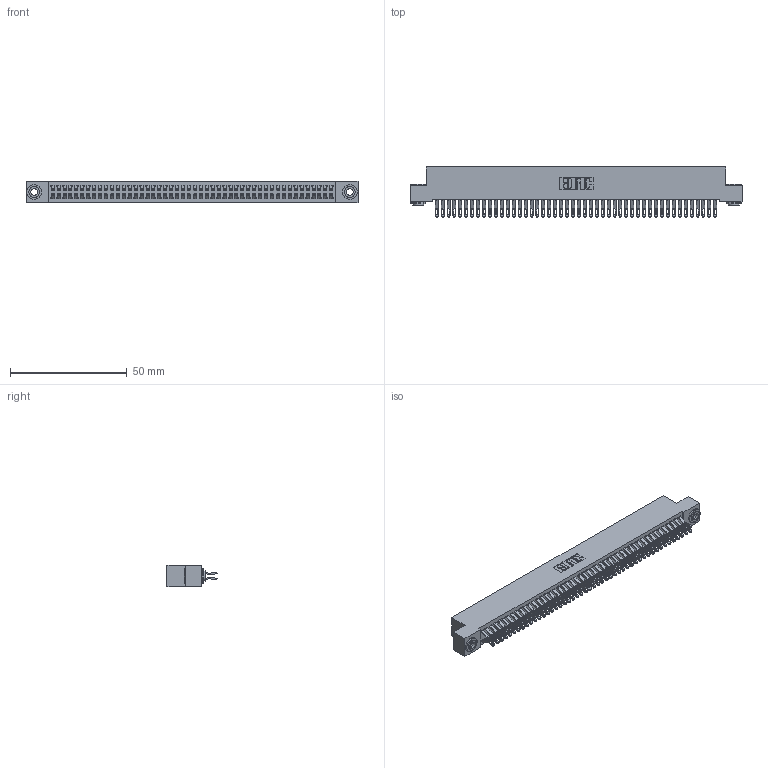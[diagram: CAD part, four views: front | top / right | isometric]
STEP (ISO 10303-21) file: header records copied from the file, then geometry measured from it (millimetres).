
FILE_DESCRIPTION (( 'STEP AP203' ), '1' );
FILE_NAME ('342-096-555-203.STEP', '2018-08-14T03:19:59', ( '' ), ( '' ), 'SwSTEP 2.0', 'SolidWorks 2016', '' );
FILE_SCHEMA (( 'CONFIG_CONTROL_DESIGN' ));
Length unit declared in the file: inch
Products named in the file (4): 342-096-555-203; 342 Part_.156 TH; 345-292-001_555 Tail; 342-250-002_345-250-002-102
Assembly tree (99 placements, depth 2):
  342-096-555-203
    342 Part_.156 TH
    345-292-001_555 Tail  x96
    342-250-002_345-250-002-102  x2
Bounding box: 142.24 x 21.47 x 9.4 mm (x, y, z)
Volume: 13098.2 mm3; surface area: 22611.4 mm2
Topology: 99 solids, 99 shells, 5716 faces, 17943 edges, 11958 vertices
Faces by surface type: plane 3340, cylinder 2368, cone 8
Entity records: 30948 total; most frequent: CARTESIAN_POINT 5131, ORIENTED_EDGE 5030, DIRECTION 4377, EDGE_CURVE 2515, LINE 2343, VECTOR 2343, VERTEX_POINT 1674, AXIS2_PLACEMENT_3D 1017
